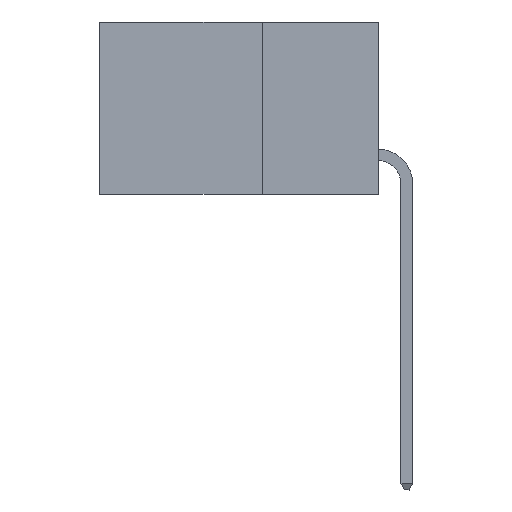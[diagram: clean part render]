
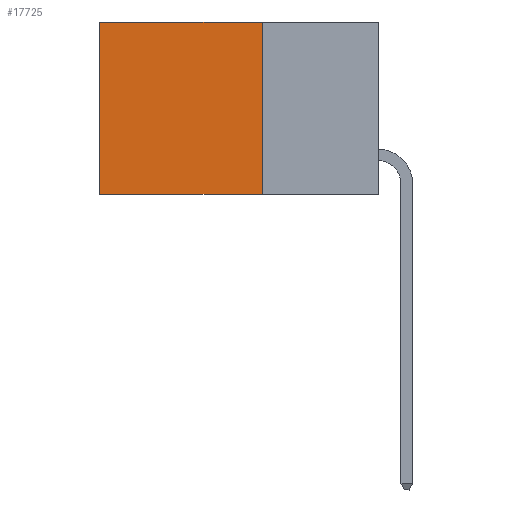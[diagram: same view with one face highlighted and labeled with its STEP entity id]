
A CAD part, left-side view. The second image highlights one B-rep face of the part: STEP entity #17725.
In plain terms, the highlighted planar face has unit normal (-1, 0, 0).
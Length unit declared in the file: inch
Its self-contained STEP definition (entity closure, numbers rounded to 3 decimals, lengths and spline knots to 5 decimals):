
#1012 = ORIENTED_EDGE ( 'NONE', *, *, #7515, .T. ) ;
#1347 = LINE ( 'NONE', #6904, #11706 ) ;
#1894 = DIRECTION ( 'NONE',  ( 0., 0., -1. ) ) ;
#2881 = VERTEX_POINT ( 'NONE', #6293 ) ;
#3229 = DIRECTION ( 'NONE',  ( 0., 0., -1. ) ) ;
#3330 = VECTOR ( 'NONE', #3229, 39.37008 ) ;
#4389 = CARTESIAN_POINT ( 'NONE',  ( 0.2615, 0.25, -0.37 ) ) ;
#4614 = CARTESIAN_POINT ( 'NONE',  ( 0.2615, 0.25, -0.37 ) ) ;
#5518 = LINE ( 'NONE', #9585, #12518 ) ;
#5692 = CARTESIAN_POINT ( 'NONE',  ( 0.2615, 0.6, -0.37 ) ) ;
#5711 = EDGE_CURVE ( 'NONE', #10680, #14468, #1347, .T. ) ;
#6293 = CARTESIAN_POINT ( 'NONE',  ( 0.2615, 0.25, -0.37 ) ) ;
#6904 = CARTESIAN_POINT ( 'NONE',  ( 0.2615, 0.6, -0.37 ) ) ;
#7395 = LINE ( 'NONE', #4614, #3330 ) ;
#7515 = EDGE_CURVE ( 'NONE', #10639, #10680, #16723, .T. ) ;
#7591 = CARTESIAN_POINT ( 'NONE',  ( 0.2615, 0.6, 0. ) ) ;
#7860 = AXIS2_PLACEMENT_3D ( 'NONE', #4389, #17074, #1894 ) ;
#9585 = CARTESIAN_POINT ( 'NONE',  ( 0.2615, 0.25, -0.37 ) ) ;
#9761 = ORIENTED_EDGE ( 'NONE', *, *, #10748, .F. ) ;
#9770 = DIRECTION ( 'NONE',  ( 0., 0., -1. ) ) ;
#10639 = VERTEX_POINT ( 'NONE', #11761 ) ;
#10680 = VERTEX_POINT ( 'NONE', #7591 ) ;
#10748 = EDGE_CURVE ( 'NONE', #10639, #2881, #7395, .T. ) ;
#10872 = ORIENTED_EDGE ( 'NONE', *, *, #5711, .T. ) ;
#11706 = VECTOR ( 'NONE', #9770, 39.37008 ) ;
#11761 = CARTESIAN_POINT ( 'NONE',  ( 0.2615, 0.25, 0. ) ) ;
#12518 = VECTOR ( 'NONE', #15336, 39.37008 ) ;
#12594 = CARTESIAN_POINT ( 'NONE',  ( 0.2615, 0.25, 0. ) ) ;
#12602 = EDGE_CURVE ( 'NONE', #2881, #14468, #5518, .T. ) ;
#13290 = FACE_OUTER_BOUND ( 'NONE', #16887, .T. ) ;
#14468 = VERTEX_POINT ( 'NONE', #5692 ) ;
#14879 = ORIENTED_EDGE ( 'NONE', *, *, #12602, .F. ) ;
#15336 = DIRECTION ( 'NONE',  ( 0., 1., 0. ) ) ;
#16204 = VECTOR ( 'NONE', #18210, 39.37008 ) ;
#16723 = LINE ( 'NONE', #12594, #16204 ) ;
#16887 = EDGE_LOOP ( 'NONE', ( #10872, #14879, #9761, #1012 ) ) ;
#17074 = DIRECTION ( 'NONE',  ( 1., 0., 0. ) ) ;
#17250 = PLANE ( 'NONE',  #7860 ) ;
#17725 = ADVANCED_FACE ( 'NONE', ( #13290 ), #17250, .F. ) ;
#18210 = DIRECTION ( 'NONE',  ( 0., 1., 0. ) ) ;
